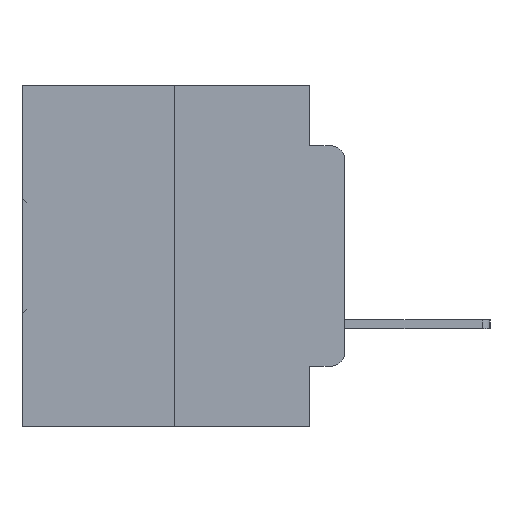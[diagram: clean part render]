
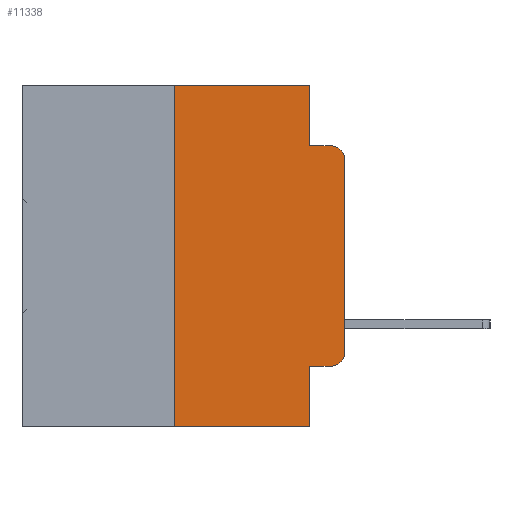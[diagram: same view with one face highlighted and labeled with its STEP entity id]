
A CAD part, left-side view. The second image highlights one B-rep face of the part: STEP entity #11338.
In plain terms, the highlighted planar face has unit normal (-1, 0, 0).
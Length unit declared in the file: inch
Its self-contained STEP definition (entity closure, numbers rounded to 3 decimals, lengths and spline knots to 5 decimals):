
#1226 = VERTEX_POINT ( 'NONE', #16716 ) ;
#1560 = CARTESIAN_POINT ( 'NONE',  ( 0., 0.02, -0.3915 ) ) ;
#1788 = DIRECTION ( 'NONE',  ( 0., 0., 1. ) ) ;
#1956 = ORIENTED_EDGE ( 'NONE', *, *, #8780, .F. ) ;
#2335 = CIRCLE ( 'NONE', #5950, 0.02 ) ;
#2643 = VERTEX_POINT ( 'NONE', #2981 ) ;
#2745 = LINE ( 'NONE', #21955, #27695 ) ;
#2981 = CARTESIAN_POINT ( 'NONE',  ( 0., 0.051, -0.5 ) ) ;
#3905 = ORIENTED_EDGE ( 'NONE', *, *, #29027, .F. ) ;
#4037 = DIRECTION ( 'NONE',  ( 0., 0., -1. ) ) ;
#4132 = DIRECTION ( 'NONE',  ( 0., 0., -1. ) ) ;
#4287 = ORIENTED_EDGE ( 'NONE', *, *, #12829, .T. ) ;
#5495 = DIRECTION ( 'NONE',  ( -1., 0., 0. ) ) ;
#5505 = EDGE_CURVE ( 'NONE', #24929, #9399, #17724, .T. ) ;
#5513 = LINE ( 'NONE', #24860, #23291 ) ;
#5769 = CARTESIAN_POINT ( 'NONE',  ( 0., 0.051, -0.4115 ) ) ;
#5950 = AXIS2_PLACEMENT_3D ( 'NONE', #19991, #5495, #22396 ) ;
#5959 = VERTEX_POINT ( 'NONE', #5769 ) ;
#6065 = VERTEX_POINT ( 'NONE', #6318 ) ;
#6098 = EDGE_CURVE ( 'NONE', #16830, #2643, #21079, .T. ) ;
#6160 = EDGE_CURVE ( 'NONE', #1226, #16958, #25948, .T. ) ;
#6318 = CARTESIAN_POINT ( 'NONE',  ( 0., 0.02, -0.4115 ) ) ;
#7394 = CIRCLE ( 'NONE', #11044, 0.02 ) ;
#8780 = EDGE_CURVE ( 'NONE', #16830, #13273, #15526, .T. ) ;
#8925 = CARTESIAN_POINT ( 'NONE',  ( 0., 0., -0.1085 ) ) ;
#9159 = DIRECTION ( 'NONE',  ( 0., -1., 0. ) ) ;
#9399 = VERTEX_POINT ( 'NONE', #29750 ) ;
#10679 = VERTEX_POINT ( 'NONE', #10729 ) ;
#10729 = CARTESIAN_POINT ( 'NONE',  ( 0., 0.051, 0. ) ) ;
#11044 = AXIS2_PLACEMENT_3D ( 'NONE', #1560, #18574, #4037 ) ;
#11072 = EDGE_CURVE ( 'NONE', #10679, #24929, #5513, .T. ) ;
#11262 = CARTESIAN_POINT ( 'NONE',  ( 0., 0.473, 0. ) ) ;
#11338 = ADVANCED_FACE ( 'NONE', ( #27752 ), #13847, .F. ) ;
#11374 = VECTOR ( 'NONE', #9159, 39.37008 ) ;
#12219 = EDGE_CURVE ( 'NONE', #5959, #2643, #2745, .T. ) ;
#12427 = DIRECTION ( 'NONE',  ( 0., 0., -1. ) ) ;
#12829 = EDGE_CURVE ( 'NONE', #5959, #6065, #17524, .T. ) ;
#13273 = VERTEX_POINT ( 'NONE', #16453 ) ;
#13778 = DIRECTION ( 'NONE',  ( 0., -1., 0. ) ) ;
#13847 = PLANE ( 'NONE',  #24468 ) ;
#13954 = VECTOR ( 'NONE', #13778, 39.37008 ) ;
#15328 = ORIENTED_EDGE ( 'NONE', *, *, #28131, .T. ) ;
#15337 = DIRECTION ( 'NONE',  ( 0., 0., -1. ) ) ;
#15526 = LINE ( 'NONE', #22261, #27514 ) ;
#15628 = EDGE_CURVE ( 'NONE', #6065, #1226, #7394, .T. ) ;
#15689 = ORIENTED_EDGE ( 'NONE', *, *, #11072, .F. ) ;
#16268 = CARTESIAN_POINT ( 'NONE',  ( 0., 0.473, 0. ) ) ;
#16453 = CARTESIAN_POINT ( 'NONE',  ( 0., 0.25, 0. ) ) ;
#16716 = CARTESIAN_POINT ( 'NONE',  ( 0., 0., -0.3915 ) ) ;
#16726 = ORIENTED_EDGE ( 'NONE', *, *, #15628, .T. ) ;
#16774 = ORIENTED_EDGE ( 'NONE', *, *, #5505, .F. ) ;
#16830 = VERTEX_POINT ( 'NONE', #30003 ) ;
#16958 = VERTEX_POINT ( 'NONE', #8925 ) ;
#17524 = LINE ( 'NONE', #21812, #29507 ) ;
#17724 = LINE ( 'NONE', #30629, #11374 ) ;
#17936 = EDGE_LOOP ( 'NONE', ( #22798, #15328, #16774, #15689, #3905, #1956, #26558, #22075, #4287, #16726 ) ) ;
#18480 = DIRECTION ( 'NONE',  ( 0., -1., 0. ) ) ;
#18574 = DIRECTION ( 'NONE',  ( -1., 0., 0. ) ) ;
#18662 = DIRECTION ( 'NONE',  ( 1., 0., 0. ) ) ;
#18784 = CARTESIAN_POINT ( 'NONE',  ( 0., 0., 0. ) ) ;
#18815 = VECTOR ( 'NONE', #1788, 39.37008 ) ;
#19364 = VECTOR ( 'NONE', #18480, 39.37008 ) ;
#19991 = CARTESIAN_POINT ( 'NONE',  ( 0., 0.02, -0.1085 ) ) ;
#21079 = LINE ( 'NONE', #23316, #13954 ) ;
#21812 = CARTESIAN_POINT ( 'NONE',  ( 0., 0.051, -0.4115 ) ) ;
#21955 = CARTESIAN_POINT ( 'NONE',  ( 0., 0.051, 0. ) ) ;
#22075 = ORIENTED_EDGE ( 'NONE', *, *, #12219, .F. ) ;
#22261 = CARTESIAN_POINT ( 'NONE',  ( 0., 0.25, 0. ) ) ;
#22396 = DIRECTION ( 'NONE',  ( 0., 0., -1. ) ) ;
#22798 = ORIENTED_EDGE ( 'NONE', *, *, #6160, .T. ) ;
#23291 = VECTOR ( 'NONE', #15337, 39.37008 ) ;
#23316 = CARTESIAN_POINT ( 'NONE',  ( 0., 0.473, -0.5 ) ) ;
#24220 = DIRECTION ( 'NONE',  ( 0., -1., 0. ) ) ;
#24468 = AXIS2_PLACEMENT_3D ( 'NONE', #16268, #18662, #4132 ) ;
#24860 = CARTESIAN_POINT ( 'NONE',  ( 0., 0.051, 0. ) ) ;
#24929 = VERTEX_POINT ( 'NONE', #25032 ) ;
#25032 = CARTESIAN_POINT ( 'NONE',  ( 0., 0.051, -0.0885 ) ) ;
#25749 = LINE ( 'NONE', #11262, #19364 ) ;
#25948 = LINE ( 'NONE', #18784, #18815 ) ;
#26558 = ORIENTED_EDGE ( 'NONE', *, *, #6098, .T. ) ;
#27514 = VECTOR ( 'NONE', #29370, 39.37008 ) ;
#27695 = VECTOR ( 'NONE', #12427, 39.37008 ) ;
#27752 = FACE_OUTER_BOUND ( 'NONE', #17936, .T. ) ;
#28131 = EDGE_CURVE ( 'NONE', #16958, #9399, #2335, .T. ) ;
#29027 = EDGE_CURVE ( 'NONE', #13273, #10679, #25749, .T. ) ;
#29370 = DIRECTION ( 'NONE',  ( 0., 0., 1. ) ) ;
#29507 = VECTOR ( 'NONE', #24220, 39.37008 ) ;
#29750 = CARTESIAN_POINT ( 'NONE',  ( 0., 0.02, -0.0885 ) ) ;
#30003 = CARTESIAN_POINT ( 'NONE',  ( 0., 0.25, -0.5 ) ) ;
#30629 = CARTESIAN_POINT ( 'NONE',  ( 0., 0.051, -0.0885 ) ) ;
